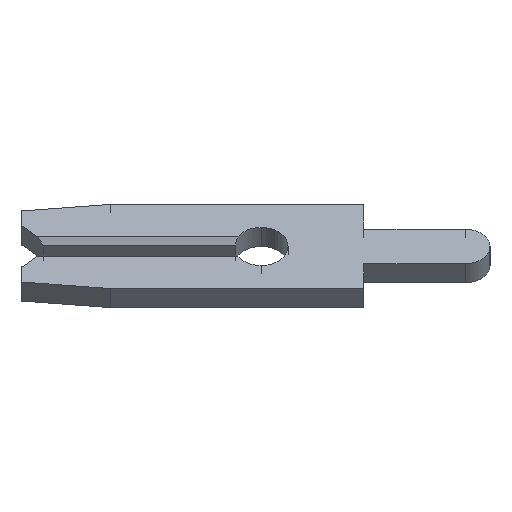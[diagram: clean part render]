
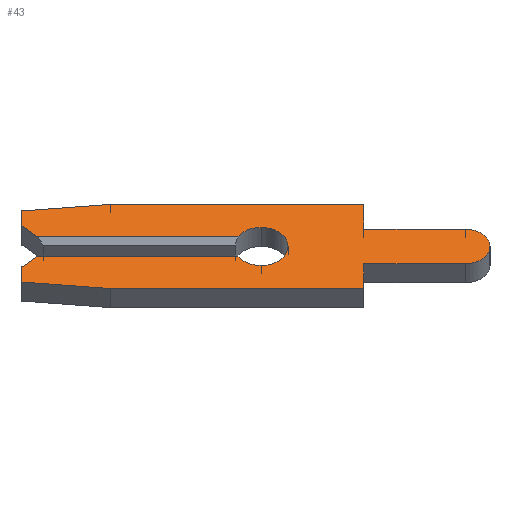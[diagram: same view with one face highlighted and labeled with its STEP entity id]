
A CAD part, left-side view. The second image highlights one B-rep face of the part: STEP entity #43.
In plain terms, the highlighted face is planar.
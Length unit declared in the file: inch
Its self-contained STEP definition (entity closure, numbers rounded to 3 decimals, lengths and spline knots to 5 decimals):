
#5 = VECTOR ( 'NONE', #1413, 39.37008 ) ;
#6 = VERTEX_POINT ( 'NONE', #1042 ) ;
#24 = VERTEX_POINT ( 'NONE', #524 ) ;
#29 = ORIENTED_EDGE ( 'NONE', *, *, #1609, .F. ) ;
#30 = LINE ( 'NONE', #1555, #692 ) ;
#35 = CARTESIAN_POINT ( 'NONE',  ( -0.013, 0., -0.013 ) ) ;
#41 = VERTEX_POINT ( 'NONE', #139 ) ;
#42 = AXIS2_PLACEMENT_3D ( 'NONE', #656, #1035, #1535 ) ;
#43 = ADVANCED_FACE ( 'NONE', ( #1521 ), #280, .F. ) ;
#45 = VECTOR ( 'NONE', #236, 39.37008 ) ;
#52 = EDGE_CURVE ( 'NONE', #753, #1077, #325, .T. ) ;
#56 = DIRECTION ( 'NONE',  ( 0., 0., 1. ) ) ;
#68 = VECTOR ( 'NONE', #1421, 39.37008 ) ;
#112 = LINE ( 'NONE', #680, #1242 ) ;
#113 = ORIENTED_EDGE ( 'NONE', *, *, #1049, .F. ) ;
#120 = EDGE_CURVE ( 'NONE', #1146, #1185, #168, .T. ) ;
#138 = EDGE_CURVE ( 'NONE', #1212, #1414, #459, .T. ) ;
#139 = CARTESIAN_POINT ( 'NONE',  ( -0.013, 0.146, 0.0575 ) ) ;
#140 = VERTEX_POINT ( 'NONE', #409 ) ;
#145 = ORIENTED_EDGE ( 'NONE', *, *, #1591, .F. ) ;
#158 = EDGE_CURVE ( 'NONE', #663, #1414, #112, .T. ) ;
#167 = EDGE_CURVE ( 'NONE', #185, #753, #1000, .T. ) ;
#168 = LINE ( 'NONE', #1405, #792 ) ;
#170 = DIRECTION ( 'NONE',  ( 0., 0.707, 0.707 ) ) ;
#185 = VERTEX_POINT ( 'NONE', #1567 ) ;
#194 = ORIENTED_EDGE ( 'NONE', *, *, #120, .F. ) ;
#200 = LINE ( 'NONE', #1313, #830 ) ;
#219 = CARTESIAN_POINT ( 'NONE',  ( -0.013, 0., 0. ) ) ;
#236 = DIRECTION ( 'NONE',  ( 0., -0.707, 0.707 ) ) ;
#280 = PLANE ( 'NONE',  #1312 ) ;
#284 = ORIENTED_EDGE ( 'NONE', *, *, #803, .F. ) ;
#290 = ORIENTED_EDGE ( 'NONE', *, *, #167, .F. ) ;
#310 = VECTOR ( 'NONE', #1540, 39.37008 ) ;
#316 = LINE ( 'NONE', #1270, #310 ) ;
#325 = LINE ( 'NONE', #1532, #68 ) ;
#330 = CARTESIAN_POINT ( 'NONE',  ( -0.013, 0., 0. ) ) ;
#363 = ORIENTED_EDGE ( 'NONE', *, *, #415, .F. ) ;
#367 = EDGE_CURVE ( 'NONE', #1243, #6, #200, .T. ) ;
#370 = VERTEX_POINT ( 'NONE', #1181 ) ;
#394 = DIRECTION ( 'NONE',  ( 0., 0., 1. ) ) ;
#405 = ORIENTED_EDGE ( 'NONE', *, *, #1225, .F. ) ;
#409 = CARTESIAN_POINT ( 'NONE',  ( -0.013, 0.02252, -0.013 ) ) ;
#415 = EDGE_CURVE ( 'NONE', #41, #185, #1382, .T. ) ;
#423 = VECTOR ( 'NONE', #1070, 39.37008 ) ;
#448 = CARTESIAN_POINT ( 'NONE',  ( -0.013, 0.02252, 0.013 ) ) ;
#455 = VERTEX_POINT ( 'NONE', #1464 ) ;
#459 = CIRCLE ( 'NONE', #42, 0.026 ) ;
#460 = CARTESIAN_POINT ( 'NONE',  ( -0.013, 0.146, -0.0575 ) ) ;
#466 = DIRECTION ( 'NONE',  ( 0., 0., -1. ) ) ;
#504 = AXIS2_PLACEMENT_3D ( 'NONE', #330, #1208, #466 ) ;
#509 = DIRECTION ( 'NONE',  ( 0., 0., -1. ) ) ;
#510 = EDGE_LOOP ( 'NONE', ( #1023, #1467, #789, #29, #802, #284, #600, #1230, #405, #1141, #145, #1333, #1302, #290, #363, #113, #194, #1558 ) ) ;
#517 = VECTOR ( 'NONE', #817, 39.37008 ) ;
#518 = VERTEX_POINT ( 'NONE', #460 ) ;
#524 = CARTESIAN_POINT ( 'NONE',  ( -0.013, 0., -0.026 ) ) ;
#528 = DIRECTION ( 'NONE',  ( 0., 0., 1. ) ) ;
#534 = CARTESIAN_POINT ( 'NONE',  ( -0.013, 0.231, 0.028 ) ) ;
#543 = CARTESIAN_POINT ( 'NONE',  ( -0.013, -0.1975, 0. ) ) ;
#551 = VECTOR ( 'NONE', #932, 39.37008 ) ;
#556 = AXIS2_PLACEMENT_3D ( 'NONE', #543, #564, #56 ) ;
#557 = CARTESIAN_POINT ( 'NONE',  ( -0.013, 0.146, -0.0575 ) ) ;
#559 = EDGE_CURVE ( 'NONE', #518, #455, #758, .T. ) ;
#564 = DIRECTION ( 'NONE',  ( 1., 0., 0. ) ) ;
#600 = ORIENTED_EDGE ( 'NONE', *, *, #987, .F. ) ;
#620 = DIRECTION ( 'NONE',  ( 0., 0., -1. ) ) ;
#639 = CARTESIAN_POINT ( 'NONE',  ( -0.013, -0.1975, 0.0235 ) ) ;
#656 = CARTESIAN_POINT ( 'NONE',  ( -0.013, 0., 0. ) ) ;
#663 = VERTEX_POINT ( 'NONE', #1463 ) ;
#676 = CARTESIAN_POINT ( 'NONE',  ( -0.013, -0.099, 0.0235 ) ) ;
#680 = CARTESIAN_POINT ( 'NONE',  ( -0.013, 0.231, 0.013 ) ) ;
#689 = DIRECTION ( 'NONE',  ( 0., -1., 0. ) ) ;
#692 = VECTOR ( 'NONE', #528, 39.37008 ) ;
#730 = VERTEX_POINT ( 'NONE', #1369 ) ;
#753 = VERTEX_POINT ( 'NONE', #676 ) ;
#755 = AXIS2_PLACEMENT_3D ( 'NONE', #219, #857, #620 ) ;
#758 = LINE ( 'NONE', #1602, #423 ) ;
#778 = EDGE_CURVE ( 'NONE', #24, #1212, #1012, .T. ) ;
#789 = ORIENTED_EDGE ( 'NONE', *, *, #778, .F. ) ;
#792 = VECTOR ( 'NONE', #394, 39.37008 ) ;
#796 = DIRECTION ( 'NONE',  ( 0., 0., -1. ) ) ;
#802 = ORIENTED_EDGE ( 'NONE', *, *, #1138, .F. ) ;
#803 = EDGE_CURVE ( 'NONE', #1205, #730, #929, .T. ) ;
#817 = DIRECTION ( 'NONE',  ( 0., -1., 0. ) ) ;
#824 = CARTESIAN_POINT ( 'NONE',  ( -0.013, 0.146, 0.0575 ) ) ;
#830 = VECTOR ( 'NONE', #796, 39.37008 ) ;
#857 = DIRECTION ( 'NONE',  ( -1., 0., 0. ) ) ;
#868 = LINE ( 'NONE', #557, #551 ) ;
#892 = CARTESIAN_POINT ( 'NONE',  ( -0.013, 0.2105, -0.0075 ) ) ;
#908 = DIRECTION ( 'NONE',  ( 0., -1., 0. ) ) ;
#926 = CARTESIAN_POINT ( 'NONE',  ( -0.013, 0.2105, 0.0075 ) ) ;
#929 = LINE ( 'NONE', #892, #45 ) ;
#932 = DIRECTION ( 'NONE',  ( 0., 1., 0. ) ) ;
#965 = DIRECTION ( 'NONE',  ( 0., 1., 0. ) ) ;
#987 = EDGE_CURVE ( 'NONE', #455, #1205, #30, .T. ) ;
#1000 = LINE ( 'NONE', #1290, #5 ) ;
#1012 = CIRCLE ( 'NONE', #755, 0.026 ) ;
#1023 = ORIENTED_EDGE ( 'NONE', *, *, #158, .T. ) ;
#1035 = DIRECTION ( 'NONE',  ( -1., 0., 0. ) ) ;
#1042 = CARTESIAN_POINT ( 'NONE',  ( -0.013, -0.099, -0.0575 ) ) ;
#1049 = EDGE_CURVE ( 'NONE', #1185, #41, #316, .T. ) ;
#1070 = DIRECTION ( 'NONE',  ( 0., 0.995, 0.105 ) ) ;
#1077 = VERTEX_POINT ( 'NONE', #639 ) ;
#1138 = EDGE_CURVE ( 'NONE', #730, #140, #1292, .T. ) ;
#1141 = ORIENTED_EDGE ( 'NONE', *, *, #367, .F. ) ;
#1146 = VERTEX_POINT ( 'NONE', #534 ) ;
#1150 = CARTESIAN_POINT ( 'NONE',  ( -0.013, 0., 0. ) ) ;
#1175 = CARTESIAN_POINT ( 'NONE',  ( -0.013, 0.231, -0.028 ) ) ;
#1181 = CARTESIAN_POINT ( 'NONE',  ( -0.013, -0.1975, -0.0235 ) ) ;
#1183 = CIRCLE ( 'NONE', #556, 0.0235 ) ;
#1185 = VERTEX_POINT ( 'NONE', #1579 ) ;
#1205 = VERTEX_POINT ( 'NONE', #1175 ) ;
#1208 = DIRECTION ( 'NONE',  ( -1., 0., 0. ) ) ;
#1212 = VERTEX_POINT ( 'NONE', #1311 ) ;
#1225 = EDGE_CURVE ( 'NONE', #6, #518, #868, .T. ) ;
#1228 = CARTESIAN_POINT ( 'NONE',  ( -0.013, -0.099, -0.0235 ) ) ;
#1229 = LINE ( 'NONE', #926, #1529 ) ;
#1230 = ORIENTED_EDGE ( 'NONE', *, *, #559, .F. ) ;
#1242 = VECTOR ( 'NONE', #689, 39.37008 ) ;
#1243 = VERTEX_POINT ( 'NONE', #1446 ) ;
#1270 = CARTESIAN_POINT ( 'NONE',  ( -0.013, 0.231, 0.04857 ) ) ;
#1290 = CARTESIAN_POINT ( 'NONE',  ( -0.013, -0.099, 0.0575 ) ) ;
#1292 = LINE ( 'NONE', #35, #1394 ) ;
#1302 = ORIENTED_EDGE ( 'NONE', *, *, #52, .F. ) ;
#1304 = EDGE_CURVE ( 'NONE', #1077, #370, #1183, .T. ) ;
#1306 = CIRCLE ( 'NONE', #504, 0.026 ) ;
#1311 = CARTESIAN_POINT ( 'NONE',  ( -0.013, 0., 0.026 ) ) ;
#1312 = AXIS2_PLACEMENT_3D ( 'NONE', #1150, #1542, #509 ) ;
#1313 = CARTESIAN_POINT ( 'NONE',  ( -0.013, -0.099, -0.0575 ) ) ;
#1333 = ORIENTED_EDGE ( 'NONE', *, *, #1304, .F. ) ;
#1369 = CARTESIAN_POINT ( 'NONE',  ( -0.013, 0.216, -0.013 ) ) ;
#1382 = LINE ( 'NONE', #824, #517 ) ;
#1392 = EDGE_CURVE ( 'NONE', #663, #1146, #1229, .T. ) ;
#1394 = VECTOR ( 'NONE', #908, 39.37008 ) ;
#1405 = CARTESIAN_POINT ( 'NONE',  ( -0.013, 0.231, 0.028 ) ) ;
#1413 = DIRECTION ( 'NONE',  ( 0., 0., -1. ) ) ;
#1414 = VERTEX_POINT ( 'NONE', #448 ) ;
#1421 = DIRECTION ( 'NONE',  ( 0., -1., 0. ) ) ;
#1439 = VECTOR ( 'NONE', #965, 39.37008 ) ;
#1446 = CARTESIAN_POINT ( 'NONE',  ( -0.013, -0.099, -0.0235 ) ) ;
#1463 = CARTESIAN_POINT ( 'NONE',  ( -0.013, 0.216, 0.013 ) ) ;
#1464 = CARTESIAN_POINT ( 'NONE',  ( -0.013, 0.231, -0.04857 ) ) ;
#1467 = ORIENTED_EDGE ( 'NONE', *, *, #138, .F. ) ;
#1521 = FACE_OUTER_BOUND ( 'NONE', #510, .T. ) ;
#1529 = VECTOR ( 'NONE', #170, 39.37008 ) ;
#1532 = CARTESIAN_POINT ( 'NONE',  ( -0.013, -0.099, 0.0235 ) ) ;
#1535 = DIRECTION ( 'NONE',  ( 0., 0., -1. ) ) ;
#1540 = DIRECTION ( 'NONE',  ( 0., -0.995, 0.105 ) ) ;
#1542 = DIRECTION ( 'NONE',  ( 1., 0., 0. ) ) ;
#1555 = CARTESIAN_POINT ( 'NONE',  ( -0.013, 0.231, -0.028 ) ) ;
#1558 = ORIENTED_EDGE ( 'NONE', *, *, #1392, .F. ) ;
#1567 = CARTESIAN_POINT ( 'NONE',  ( -0.013, -0.099, 0.0575 ) ) ;
#1579 = CARTESIAN_POINT ( 'NONE',  ( -0.013, 0.231, 0.04857 ) ) ;
#1591 = EDGE_CURVE ( 'NONE', #370, #1243, #1596, .T. ) ;
#1596 = LINE ( 'NONE', #1228, #1439 ) ;
#1602 = CARTESIAN_POINT ( 'NONE',  ( -0.013, 0.231, -0.04857 ) ) ;
#1609 = EDGE_CURVE ( 'NONE', #140, #24, #1306, .T. ) ;
